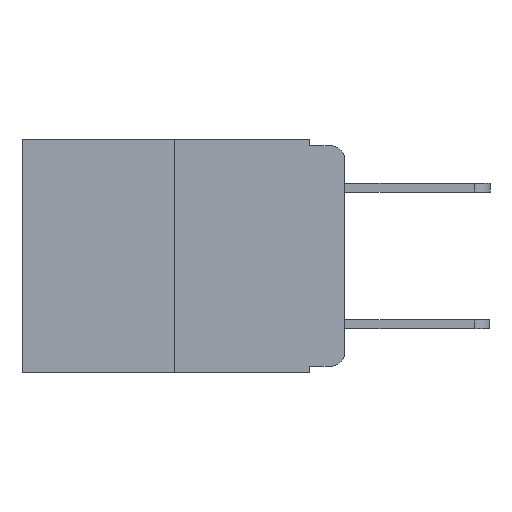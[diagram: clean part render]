
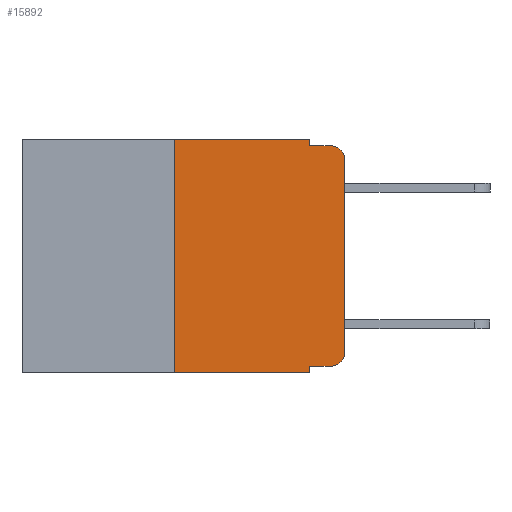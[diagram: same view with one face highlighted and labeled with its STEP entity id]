
A CAD part, left-side view. The second image highlights one B-rep face of the part: STEP entity #15892.
In plain terms, the highlighted planar face has unit normal (-1, 0, 0).
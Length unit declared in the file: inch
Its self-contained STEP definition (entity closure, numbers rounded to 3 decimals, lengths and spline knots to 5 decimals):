
#169 = CARTESIAN_POINT ( 'NONE',  ( 0., 0.02, -0.313 ) ) ;
#197 = EDGE_LOOP ( 'NONE', ( #13952, #14757, #5290, #10203, #12268, #4527, #6178, #17152, #12775, #17436 ) ) ;
#240 = CARTESIAN_POINT ( 'NONE',  ( 0., 0.25, -0.343 ) ) ;
#465 = CARTESIAN_POINT ( 'NONE',  ( 0., 0.02, -0.333 ) ) ;
#855 = VERTEX_POINT ( 'NONE', #465 ) ;
#978 = LINE ( 'NONE', #5241, #5054 ) ;
#1035 = DIRECTION ( 'NONE',  ( 0., 0., 1. ) ) ;
#1202 = LINE ( 'NONE', #5190, #4427 ) ;
#1368 = DIRECTION ( 'NONE',  ( 0., 0., -1. ) ) ;
#1602 = EDGE_CURVE ( 'NONE', #8048, #2000, #11489, .T. ) ;
#1606 = VECTOR ( 'NONE', #16890, 39.37008 ) ;
#1839 = EDGE_CURVE ( 'NONE', #2000, #12105, #1202, .T. ) ;
#1970 = CARTESIAN_POINT ( 'NONE',  ( 0., 0.051, -0.333 ) ) ;
#2000 = VERTEX_POINT ( 'NONE', #3704 ) ;
#2279 = PLANE ( 'NONE',  #17243 ) ;
#2844 = EDGE_CURVE ( 'NONE', #855, #10630, #10369, .T. ) ;
#3123 = VECTOR ( 'NONE', #14360, 39.37008 ) ;
#3184 = CARTESIAN_POINT ( 'NONE',  ( 0., 0., 0. ) ) ;
#3245 = DIRECTION ( 'NONE',  ( -1., 0., 0. ) ) ;
#3704 = CARTESIAN_POINT ( 'NONE',  ( 0., 0.051, -0.01 ) ) ;
#3872 = DIRECTION ( 'NONE',  ( -1., 0., 0. ) ) ;
#4427 = VECTOR ( 'NONE', #6510, 39.37008 ) ;
#4527 = ORIENTED_EDGE ( 'NONE', *, *, #8348, .F. ) ;
#5054 = VECTOR ( 'NONE', #1035, 39.37008 ) ;
#5141 = EDGE_CURVE ( 'NONE', #7110, #855, #16758, .T. ) ;
#5190 = CARTESIAN_POINT ( 'NONE',  ( 0., 0.051, -0.01 ) ) ;
#5241 = CARTESIAN_POINT ( 'NONE',  ( 0., 0.25, 0. ) ) ;
#5290 = ORIENTED_EDGE ( 'NONE', *, *, #1839, .F. ) ;
#6170 = VERTEX_POINT ( 'NONE', #9657 ) ;
#6178 = ORIENTED_EDGE ( 'NONE', *, *, #14134, .T. ) ;
#6391 = CARTESIAN_POINT ( 'NONE',  ( 0., 0.473, 0. ) ) ;
#6510 = DIRECTION ( 'NONE',  ( 0., -1., 0. ) ) ;
#6743 = LINE ( 'NONE', #13008, #3123 ) ;
#7110 = VERTEX_POINT ( 'NONE', #17264 ) ;
#7703 = CARTESIAN_POINT ( 'NONE',  ( 0., 0.473, -0.343 ) ) ;
#7762 = DIRECTION ( 'NONE',  ( 0., 0., -1. ) ) ;
#7889 = VECTOR ( 'NONE', #15360, 39.37008 ) ;
#8048 = VERTEX_POINT ( 'NONE', #11337 ) ;
#8257 = VECTOR ( 'NONE', #12814, 39.37008 ) ;
#8293 = LINE ( 'NONE', #16760, #7889 ) ;
#8332 = EDGE_CURVE ( 'NONE', #6170, #12105, #12346, .T. ) ;
#8348 = EDGE_CURVE ( 'NONE', #11913, #9048, #978, .T. ) ;
#8826 = CARTESIAN_POINT ( 'NONE',  ( 0., 0.02, -0.01 ) ) ;
#8841 = LINE ( 'NONE', #7703, #15729 ) ;
#9048 = VERTEX_POINT ( 'NONE', #13027 ) ;
#9057 = DIRECTION ( 'NONE',  ( 0., -1., 0. ) ) ;
#9452 = FACE_OUTER_BOUND ( 'NONE', #197, .T. ) ;
#9506 = EDGE_CURVE ( 'NONE', #10630, #6170, #16635, .T. ) ;
#9630 = EDGE_CURVE ( 'NONE', #9048, #8048, #6743, .T. ) ;
#9657 = CARTESIAN_POINT ( 'NONE',  ( 0., 0., -0.03 ) ) ;
#9685 = AXIS2_PLACEMENT_3D ( 'NONE', #12071, #3872, #13463 ) ;
#10147 = DIRECTION ( 'NONE',  ( 0., -1., 0. ) ) ;
#10203 = ORIENTED_EDGE ( 'NONE', *, *, #1602, .F. ) ;
#10369 = CIRCLE ( 'NONE', #16199, 0.02 ) ;
#10630 = VERTEX_POINT ( 'NONE', #12554 ) ;
#11337 = CARTESIAN_POINT ( 'NONE',  ( 0., 0.051, 0. ) ) ;
#11489 = LINE ( 'NONE', #11616, #8257 ) ;
#11604 = CARTESIAN_POINT ( 'NONE',  ( 0., 0.051, -0.343 ) ) ;
#11616 = CARTESIAN_POINT ( 'NONE',  ( 0., 0.051, 0. ) ) ;
#11913 = VERTEX_POINT ( 'NONE', #240 ) ;
#12071 = CARTESIAN_POINT ( 'NONE',  ( 0., 0.02, -0.03 ) ) ;
#12105 = VERTEX_POINT ( 'NONE', #8826 ) ;
#12268 = ORIENTED_EDGE ( 'NONE', *, *, #9630, .F. ) ;
#12346 = CIRCLE ( 'NONE', #9685, 0.02 ) ;
#12554 = CARTESIAN_POINT ( 'NONE',  ( 0., 0., -0.313 ) ) ;
#12775 = ORIENTED_EDGE ( 'NONE', *, *, #5141, .T. ) ;
#12814 = DIRECTION ( 'NONE',  ( 0., 0., -1. ) ) ;
#13008 = CARTESIAN_POINT ( 'NONE',  ( 0., 0.473, 0. ) ) ;
#13027 = CARTESIAN_POINT ( 'NONE',  ( 0., 0.25, 0. ) ) ;
#13114 = VECTOR ( 'NONE', #10147, 39.37008 ) ;
#13463 = DIRECTION ( 'NONE',  ( 0., 0., -1. ) ) ;
#13952 = ORIENTED_EDGE ( 'NONE', *, *, #9506, .T. ) ;
#14029 = VERTEX_POINT ( 'NONE', #11604 ) ;
#14134 = EDGE_CURVE ( 'NONE', #11913, #14029, #8841, .T. ) ;
#14360 = DIRECTION ( 'NONE',  ( 0., -1., 0. ) ) ;
#14757 = ORIENTED_EDGE ( 'NONE', *, *, #8332, .T. ) ;
#15360 = DIRECTION ( 'NONE',  ( 0., 0., -1. ) ) ;
#15729 = VECTOR ( 'NONE', #9057, 39.37008 ) ;
#15892 = ADVANCED_FACE ( 'NONE', ( #9452 ), #2279, .F. ) ;
#15978 = DIRECTION ( 'NONE',  ( 1., 0., 0. ) ) ;
#16199 = AXIS2_PLACEMENT_3D ( 'NONE', #169, #3245, #1368 ) ;
#16635 = LINE ( 'NONE', #3184, #1606 ) ;
#16758 = LINE ( 'NONE', #1970, #13114 ) ;
#16760 = CARTESIAN_POINT ( 'NONE',  ( 0., 0.051, 0. ) ) ;
#16890 = DIRECTION ( 'NONE',  ( 0., 0., 1. ) ) ;
#17152 = ORIENTED_EDGE ( 'NONE', *, *, #17725, .F. ) ;
#17243 = AXIS2_PLACEMENT_3D ( 'NONE', #6391, #15978, #7762 ) ;
#17264 = CARTESIAN_POINT ( 'NONE',  ( 0., 0.051, -0.333 ) ) ;
#17436 = ORIENTED_EDGE ( 'NONE', *, *, #2844, .T. ) ;
#17725 = EDGE_CURVE ( 'NONE', #7110, #14029, #8293, .T. ) ;
